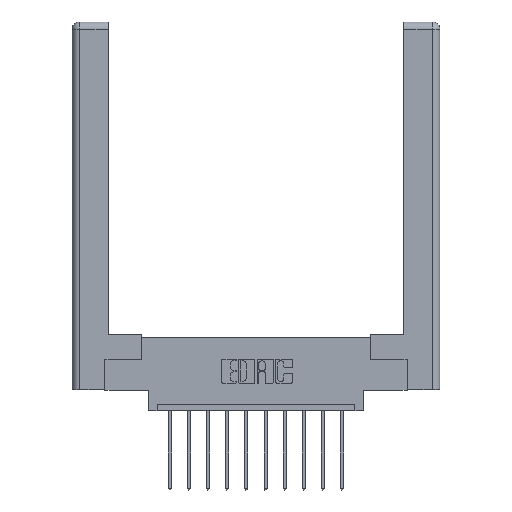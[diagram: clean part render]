
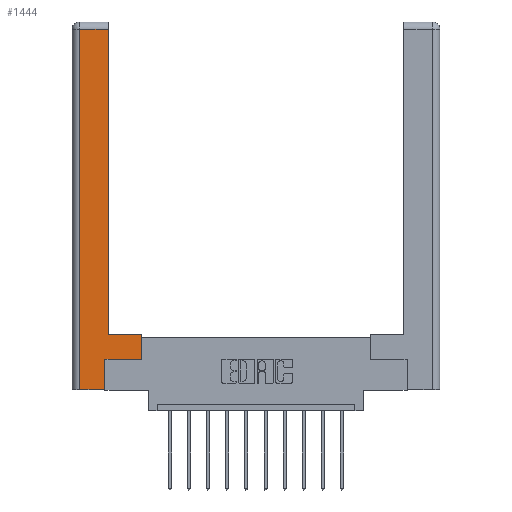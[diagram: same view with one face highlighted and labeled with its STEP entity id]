
A CAD part, top view. The second image highlights one B-rep face of the part: STEP entity #1444.
In plain terms, the highlighted planar face has unit normal (0, 0, 1).
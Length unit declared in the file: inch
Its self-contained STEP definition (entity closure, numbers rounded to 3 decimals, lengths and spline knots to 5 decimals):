
#123 = LINE ( 'NONE', #7175, #13660 ) ;
#199 = EDGE_CURVE ( 'NONE', #11990, #11520, #3328, .T. ) ;
#282 = CARTESIAN_POINT ( 'NONE',  ( 0.295, 0.45, 0. ) ) ;
#407 = VECTOR ( 'NONE', #594, 39.37008 ) ;
#418 = CARTESIAN_POINT ( 'NONE',  ( 0.295, 3., 0. ) ) ;
#527 = CARTESIAN_POINT ( 'NONE',  ( 0.0615, 2.94, 0. ) ) ;
#594 = DIRECTION ( 'NONE',  ( 1., 0., 0. ) ) ;
#805 = CARTESIAN_POINT ( 'NONE',  ( 0.565, 0.245, 0. ) ) ;
#1117 = EDGE_LOOP ( 'NONE', ( #12222, #4584, #6271, #7255, #10328, #9405, #9471, #7880 ) ) ;
#1119 = CARTESIAN_POINT ( 'NONE',  ( 0., 0., 0. ) ) ;
#1212 = CARTESIAN_POINT ( 'NONE',  ( 0.0615, 0., 0. ) ) ;
#1444 = ADVANCED_FACE ( 'NONE', ( #12154 ), #11054, .F. ) ;
#1491 = CARTESIAN_POINT ( 'NONE',  ( 0.265, 0.245, 0. ) ) ;
#2692 = VECTOR ( 'NONE', #7613, 39.37008 ) ;
#2728 = VERTEX_POINT ( 'NONE', #282 ) ;
#2771 = CARTESIAN_POINT ( 'NONE',  ( 0.0615, 2.94, 0. ) ) ;
#2879 = VECTOR ( 'NONE', #8628, 39.37008 ) ;
#3223 = EDGE_CURVE ( 'NONE', #2728, #7644, #10388, .T. ) ;
#3328 = LINE ( 'NONE', #8402, #407 ) ;
#4584 = ORIENTED_EDGE ( 'NONE', *, *, #13549, .T. ) ;
#4631 = CARTESIAN_POINT ( 'NONE',  ( 0.265, 0., 0. ) ) ;
#5694 = VECTOR ( 'NONE', #12759, 39.37008 ) ;
#5716 = VECTOR ( 'NONE', #9369, 39.37008 ) ;
#5956 = VERTEX_POINT ( 'NONE', #6215 ) ;
#6013 = DIRECTION ( 'NONE',  ( 0., 1., 0. ) ) ;
#6215 = CARTESIAN_POINT ( 'NONE',  ( 0.565, 0.45, 0. ) ) ;
#6271 = ORIENTED_EDGE ( 'NONE', *, *, #12255, .T. ) ;
#6313 = VERTEX_POINT ( 'NONE', #1212 ) ;
#6723 = LINE ( 'NONE', #11555, #5694 ) ;
#7175 = CARTESIAN_POINT ( 'NONE',  ( 0.565, 0.45, 0. ) ) ;
#7201 = VERTEX_POINT ( 'NONE', #527 ) ;
#7247 = DIRECTION ( 'NONE',  ( 1., 0., 0. ) ) ;
#7255 = ORIENTED_EDGE ( 'NONE', *, *, #7257, .T. ) ;
#7257 = EDGE_CURVE ( 'NONE', #6313, #11971, #13215, .T. ) ;
#7592 = LINE ( 'NONE', #2771, #2692 ) ;
#7613 = DIRECTION ( 'NONE',  ( -1., 0., 0. ) ) ;
#7644 = VERTEX_POINT ( 'NONE', #7857 ) ;
#7826 = CARTESIAN_POINT ( 'NONE',  ( 0.0615, 0., 0. ) ) ;
#7857 = CARTESIAN_POINT ( 'NONE',  ( 0.295, 2.94, 0. ) ) ;
#7880 = ORIENTED_EDGE ( 'NONE', *, *, #10914, .T. ) ;
#8402 = CARTESIAN_POINT ( 'NONE',  ( 0.565, 0.245, 0. ) ) ;
#8628 = DIRECTION ( 'NONE',  ( 0., 1., 0. ) ) ;
#8815 = LINE ( 'NONE', #9871, #2879 ) ;
#9369 = DIRECTION ( 'NONE',  ( 0., 1., 0. ) ) ;
#9405 = ORIENTED_EDGE ( 'NONE', *, *, #199, .T. ) ;
#9471 = ORIENTED_EDGE ( 'NONE', *, *, #10542, .T. ) ;
#9871 = CARTESIAN_POINT ( 'NONE',  ( 0.265, 0.245, 0. ) ) ;
#10117 = AXIS2_PLACEMENT_3D ( 'NONE', #1119, #10924, #10965 ) ;
#10328 = ORIENTED_EDGE ( 'NONE', *, *, #11144, .T. ) ;
#10388 = LINE ( 'NONE', #418, #5716 ) ;
#10542 = EDGE_CURVE ( 'NONE', #11520, #5956, #123, .T. ) ;
#10914 = EDGE_CURVE ( 'NONE', #5956, #2728, #6723, .T. ) ;
#10924 = DIRECTION ( 'NONE',  ( 0., 0., -1. ) ) ;
#10965 = DIRECTION ( 'NONE',  ( -1., 0., 0. ) ) ;
#10986 = VECTOR ( 'NONE', #7247, 39.37008 ) ;
#11054 = PLANE ( 'NONE',  #10117 ) ;
#11144 = EDGE_CURVE ( 'NONE', #11971, #11990, #8815, .T. ) ;
#11199 = DIRECTION ( 'NONE',  ( 0., -1., 0. ) ) ;
#11520 = VERTEX_POINT ( 'NONE', #805 ) ;
#11555 = CARTESIAN_POINT ( 'NONE',  ( 0.295, 0.45, 0. ) ) ;
#11971 = VERTEX_POINT ( 'NONE', #4631 ) ;
#11990 = VERTEX_POINT ( 'NONE', #1491 ) ;
#12154 = FACE_OUTER_BOUND ( 'NONE', #1117, .T. ) ;
#12222 = ORIENTED_EDGE ( 'NONE', *, *, #3223, .T. ) ;
#12255 = EDGE_CURVE ( 'NONE', #7201, #6313, #13310, .T. ) ;
#12740 = CARTESIAN_POINT ( 'NONE',  ( 0.265, 0., 0. ) ) ;
#12759 = DIRECTION ( 'NONE',  ( -1., 0., 0. ) ) ;
#13215 = LINE ( 'NONE', #12740, #10986 ) ;
#13310 = LINE ( 'NONE', #7826, #14202 ) ;
#13549 = EDGE_CURVE ( 'NONE', #7644, #7201, #7592, .T. ) ;
#13660 = VECTOR ( 'NONE', #6013, 39.37008 ) ;
#14202 = VECTOR ( 'NONE', #11199, 39.37008 ) ;
